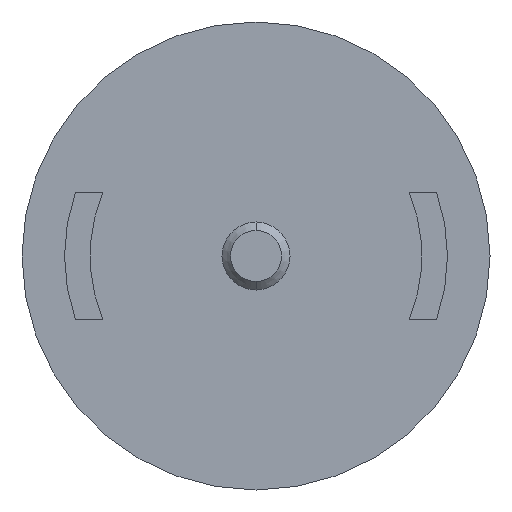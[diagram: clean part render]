
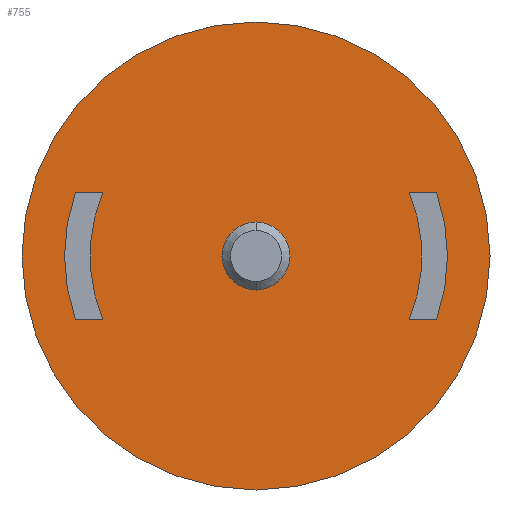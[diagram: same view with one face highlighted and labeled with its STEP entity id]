
A CAD part, front view. The second image highlights one B-rep face of the part: STEP entity #755.
In plain terms, the highlighted planar face has unit normal (0, -1, 0).
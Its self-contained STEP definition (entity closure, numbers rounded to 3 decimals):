
#13 = CARTESIAN_POINT ( 'NONE',  ( 2.121, -2.45, 0.75 ) ) ;
#97 = VECTOR ( 'NONE', #1040, 1000. ) ;
#116 = FACE_OUTER_BOUND ( 'NONE', #1137, .T. ) ;
#133 = CARTESIAN_POINT ( 'NONE',  ( 0., -2.45, 0. ) ) ;
#136 = ORIENTED_EDGE ( 'NONE', *, *, #780, .T. ) ;
#137 = LINE ( 'NONE', #1662, #1414 ) ;
#240 = CIRCLE ( 'NONE', #1487, 2.75 ) ;
#248 = ORIENTED_EDGE ( 'NONE', *, *, #289, .T. ) ;
#260 = CARTESIAN_POINT ( 'NONE',  ( 0., -2.45, 0. ) ) ;
#263 = DIRECTION ( 'NONE',  ( 0., 0., 1. ) ) ;
#265 = CARTESIAN_POINT ( 'NONE',  ( -2.121, -2.45, -0.75 ) ) ;
#289 = EDGE_CURVE ( 'NONE', #295, #475, #1563, .T. ) ;
#295 = VERTEX_POINT ( 'NONE', #1113 ) ;
#315 = VERTEX_POINT ( 'NONE', #265 ) ;
#322 = DIRECTION ( 'NONE',  ( 0., 0., 1. ) ) ;
#347 = CIRCLE ( 'NONE', #837, 0.4 ) ;
#359 = EDGE_CURVE ( 'NONE', #2046, #295, #1930, .T. ) ;
#375 = DIRECTION ( 'NONE',  ( 1., 0., 0. ) ) ;
#392 = DIRECTION ( 'NONE',  ( 1., 0., 0. ) ) ;
#414 = CARTESIAN_POINT ( 'NONE',  ( -1.8, -2.45, -0.75 ) ) ;
#419 = CIRCLE ( 'NONE', #764, 2.75 ) ;
#423 = DIRECTION ( 'NONE',  ( -0.923, 0., 0.385 ) ) ;
#474 = CARTESIAN_POINT ( 'NONE',  ( 0., -2.45, -2.75 ) ) ;
#475 = VERTEX_POINT ( 'NONE', #477 ) ;
#477 = CARTESIAN_POINT ( 'NONE',  ( 1.8, -2.45, 0.75 ) ) ;
#503 = AXIS2_PLACEMENT_3D ( 'NONE', #2181, #2019, #779 ) ;
#510 = EDGE_CURVE ( 'NONE', #605, #2046, #812, .T. ) ;
#522 = EDGE_LOOP ( 'NONE', ( #1344, #1774 ) ) ;
#577 = AXIS2_PLACEMENT_3D ( 'NONE', #260, #939, #423 ) ;
#605 = VERTEX_POINT ( 'NONE', #13 ) ;
#621 = FACE_BOUND ( 'NONE', #1362, .T. ) ;
#668 = CARTESIAN_POINT ( 'NONE',  ( 0., -2.45, 0. ) ) ;
#680 = ORIENTED_EDGE ( 'NONE', *, *, #934, .T. ) ;
#737 = CIRCLE ( 'NONE', #1705, 0.4 ) ;
#755 = ADVANCED_FACE ( 'NONE', ( #116, #621, #1488, #1290 ), #1638, .F. ) ;
#764 = AXIS2_PLACEMENT_3D ( 'NONE', #1042, #1736, #1022 ) ;
#765 = EDGE_CURVE ( 'NONE', #1498, #2170, #240, .T. ) ;
#779 = DIRECTION ( 'NONE',  ( 0.923, 0., -0.385 ) ) ;
#780 = EDGE_CURVE ( 'NONE', #315, #1286, #1670, .T. ) ;
#797 = DIRECTION ( 'NONE',  ( -1., 0., 0. ) ) ;
#812 = CIRCLE ( 'NONE', #1088, 2.25 ) ;
#837 = AXIS2_PLACEMENT_3D ( 'NONE', #133, #1859, #322 ) ;
#934 = EDGE_CURVE ( 'NONE', #475, #605, #1915, .T. ) ;
#939 = DIRECTION ( 'NONE',  ( 0., -1., 0. ) ) ;
#967 = DIRECTION ( 'NONE',  ( 0., 1., 0. ) ) ;
#987 = CARTESIAN_POINT ( 'NONE',  ( 2.121, -2.45, -0.75 ) ) ;
#999 = DIRECTION ( 'NONE',  ( -0.943, 0., -0.333 ) ) ;
#1003 = VECTOR ( 'NONE', #375, 1000. ) ;
#1011 = CARTESIAN_POINT ( 'NONE',  ( 0., -2.45, 2.75 ) ) ;
#1022 = DIRECTION ( 'NONE',  ( 0., 0., -1. ) ) ;
#1034 = CARTESIAN_POINT ( 'NONE',  ( -1.8, -2.45, 0.75 ) ) ;
#1040 = DIRECTION ( 'NONE',  ( -1., 0., 0. ) ) ;
#1042 = CARTESIAN_POINT ( 'NONE',  ( 0., -2.45, 0. ) ) ;
#1080 = AXIS2_PLACEMENT_3D ( 'NONE', #1463, #1830, #1975 ) ;
#1088 = AXIS2_PLACEMENT_3D ( 'NONE', #1499, #967, #1520 ) ;
#1090 = EDGE_CURVE ( 'NONE', #2119, #1438, #737, .T. ) ;
#1101 = CARTESIAN_POINT ( 'NONE',  ( 0., -2.45, 0. ) ) ;
#1113 = CARTESIAN_POINT ( 'NONE',  ( 1.8, -2.45, -0.75 ) ) ;
#1130 = EDGE_CURVE ( 'NONE', #1333, #315, #137, .T. ) ;
#1137 = EDGE_LOOP ( 'NONE', ( #2122, #1611 ) ) ;
#1196 = EDGE_CURVE ( 'NONE', #2170, #1498, #419, .T. ) ;
#1216 = VERTEX_POINT ( 'NONE', #1034 ) ;
#1234 = CARTESIAN_POINT ( 'NONE',  ( -2.121, -2.45, 0.75 ) ) ;
#1258 = CARTESIAN_POINT ( 'NONE',  ( 0., -2.45, -0.4 ) ) ;
#1286 = VERTEX_POINT ( 'NONE', #1383 ) ;
#1290 = FACE_BOUND ( 'NONE', #522, .T. ) ;
#1295 = DIRECTION ( 'NONE',  ( 0., 0., -1. ) ) ;
#1333 = VERTEX_POINT ( 'NONE', #414 ) ;
#1344 = ORIENTED_EDGE ( 'NONE', *, *, #2009, .F. ) ;
#1350 = DIRECTION ( 'NONE',  ( 0., 1., 0. ) ) ;
#1362 = EDGE_LOOP ( 'NONE', ( #1424, #136, #1789, #1468 ) ) ;
#1383 = CARTESIAN_POINT ( 'NONE',  ( -2.121, -2.45, 0.75 ) ) ;
#1414 = VECTOR ( 'NONE', #797, 1000. ) ;
#1424 = ORIENTED_EDGE ( 'NONE', *, *, #1130, .T. ) ;
#1438 = VERTEX_POINT ( 'NONE', #1444 ) ;
#1440 = EDGE_LOOP ( 'NONE', ( #1519, #248, #680, #1841 ) ) ;
#1444 = CARTESIAN_POINT ( 'NONE',  ( 0., -2.45, 0.4 ) ) ;
#1449 = AXIS2_PLACEMENT_3D ( 'NONE', #668, #1350, #999 ) ;
#1463 = CARTESIAN_POINT ( 'NONE',  ( 0.4, -2.45, 0. ) ) ;
#1468 = ORIENTED_EDGE ( 'NONE', *, *, #1709, .T. ) ;
#1487 = AXIS2_PLACEMENT_3D ( 'NONE', #1101, #1807, #263 ) ;
#1488 = FACE_BOUND ( 'NONE', #1440, .T. ) ;
#1498 = VERTEX_POINT ( 'NONE', #1011 ) ;
#1499 = CARTESIAN_POINT ( 'NONE',  ( 0., -2.45, 0. ) ) ;
#1513 = CARTESIAN_POINT ( 'NONE',  ( 2.121, -2.45, -0.75 ) ) ;
#1519 = ORIENTED_EDGE ( 'NONE', *, *, #359, .T. ) ;
#1520 = DIRECTION ( 'NONE',  ( 0.943, 0., 0.333 ) ) ;
#1543 = LINE ( 'NONE', #1234, #1969 ) ;
#1563 = CIRCLE ( 'NONE', #503, 1.95 ) ;
#1575 = EDGE_CURVE ( 'NONE', #1286, #1216, #1543, .T. ) ;
#1611 = ORIENTED_EDGE ( 'NONE', *, *, #1196, .T. ) ;
#1638 = PLANE ( 'NONE',  #1080 ) ;
#1662 = CARTESIAN_POINT ( 'NONE',  ( -1.8, -2.45, -0.75 ) ) ;
#1670 = CIRCLE ( 'NONE', #1449, 2.25 ) ;
#1705 = AXIS2_PLACEMENT_3D ( 'NONE', #1867, #2011, #1295 ) ;
#1709 = EDGE_CURVE ( 'NONE', #1216, #1333, #1828, .T. ) ;
#1736 = DIRECTION ( 'NONE',  ( 0., -1., 0. ) ) ;
#1756 = CARTESIAN_POINT ( 'NONE',  ( 1.8, -2.45, 0.75 ) ) ;
#1774 = ORIENTED_EDGE ( 'NONE', *, *, #1090, .F. ) ;
#1789 = ORIENTED_EDGE ( 'NONE', *, *, #1575, .T. ) ;
#1807 = DIRECTION ( 'NONE',  ( 0., -1., 0. ) ) ;
#1828 = CIRCLE ( 'NONE', #577, 1.95 ) ;
#1830 = DIRECTION ( 'NONE',  ( 0., 1., 0. ) ) ;
#1841 = ORIENTED_EDGE ( 'NONE', *, *, #510, .T. ) ;
#1859 = DIRECTION ( 'NONE',  ( 0., -1., 0. ) ) ;
#1867 = CARTESIAN_POINT ( 'NONE',  ( 0., -2.45, 0. ) ) ;
#1915 = LINE ( 'NONE', #1756, #1003 ) ;
#1930 = LINE ( 'NONE', #987, #97 ) ;
#1969 = VECTOR ( 'NONE', #392, 1000. ) ;
#1975 = DIRECTION ( 'NONE',  ( 1., 0., 0. ) ) ;
#2009 = EDGE_CURVE ( 'NONE', #1438, #2119, #347, .T. ) ;
#2011 = DIRECTION ( 'NONE',  ( 0., -1., 0. ) ) ;
#2019 = DIRECTION ( 'NONE',  ( 0., -1., 0. ) ) ;
#2046 = VERTEX_POINT ( 'NONE', #1513 ) ;
#2119 = VERTEX_POINT ( 'NONE', #1258 ) ;
#2122 = ORIENTED_EDGE ( 'NONE', *, *, #765, .T. ) ;
#2170 = VERTEX_POINT ( 'NONE', #474 ) ;
#2181 = CARTESIAN_POINT ( 'NONE',  ( 0., -2.45, 0. ) ) ;
